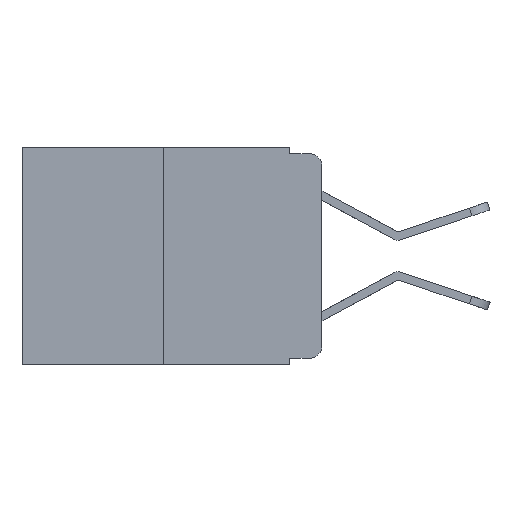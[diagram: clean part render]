
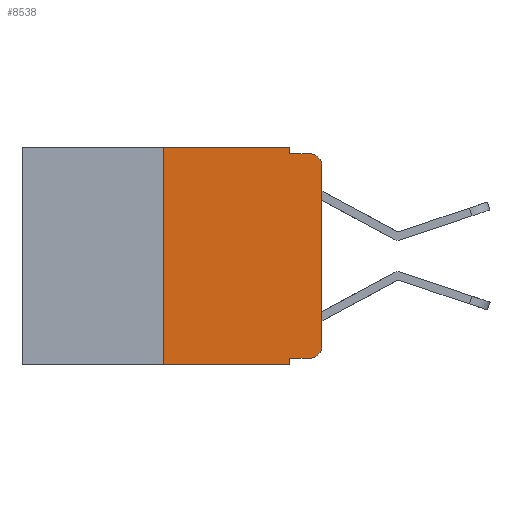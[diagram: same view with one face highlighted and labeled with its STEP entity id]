
A CAD part, left-side view. The second image highlights one B-rep face of the part: STEP entity #8538.
In plain terms, the highlighted planar face has unit normal (-1, 0, 0).
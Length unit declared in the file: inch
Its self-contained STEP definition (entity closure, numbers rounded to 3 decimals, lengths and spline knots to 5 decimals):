
#39 = EDGE_CURVE ( 'NONE', #12802, #1607, #10376, .T. ) ;
#123 = ORIENTED_EDGE ( 'NONE', *, *, #5390, .F. ) ;
#180 = ORIENTED_EDGE ( 'NONE', *, *, #4472, .F. ) ;
#557 = LINE ( 'NONE', #7894, #12925 ) ;
#596 = DIRECTION ( 'NONE',  ( 0., 0., -1. ) ) ;
#652 = LINE ( 'NONE', #930, #7725 ) ;
#930 = CARTESIAN_POINT ( 'NONE',  ( 0., 0.473, -0.343 ) ) ;
#1021 = DIRECTION ( 'NONE',  ( -1., 0., 0. ) ) ;
#1055 = EDGE_CURVE ( 'NONE', #1607, #8877, #1795, .T. ) ;
#1063 = DIRECTION ( 'NONE',  ( 0., 0., 1. ) ) ;
#1137 = CARTESIAN_POINT ( 'NONE',  ( 0., 0.051, -0.343 ) ) ;
#1158 = EDGE_CURVE ( 'NONE', #9367, #1468, #9907, .T. ) ;
#1468 = VERTEX_POINT ( 'NONE', #4644 ) ;
#1482 = VERTEX_POINT ( 'NONE', #1757 ) ;
#1556 = CARTESIAN_POINT ( 'NONE',  ( 0., 0.051, 0. ) ) ;
#1607 = VERTEX_POINT ( 'NONE', #6348 ) ;
#1757 = CARTESIAN_POINT ( 'NONE',  ( 0., 0.25, 0. ) ) ;
#1795 = CIRCLE ( 'NONE', #2024, 0.02 ) ;
#1872 = ORIENTED_EDGE ( 'NONE', *, *, #1055, .T. ) ;
#1900 = VECTOR ( 'NONE', #13041, 39.37008 ) ;
#2024 = AXIS2_PLACEMENT_3D ( 'NONE', #3216, #1021, #5986 ) ;
#2166 = CARTESIAN_POINT ( 'NONE',  ( 0., 0., 0. ) ) ;
#2425 = VERTEX_POINT ( 'NONE', #8123 ) ;
#2855 = DIRECTION ( 'NONE',  ( 0., 0., 1. ) ) ;
#3163 = AXIS2_PLACEMENT_3D ( 'NONE', #7891, #5047, #3957 ) ;
#3193 = EDGE_CURVE ( 'NONE', #12221, #12802, #10938, .T. ) ;
#3216 = CARTESIAN_POINT ( 'NONE',  ( 0., 0.02, -0.03 ) ) ;
#3220 = VECTOR ( 'NONE', #2855, 39.37008 ) ;
#3554 = DIRECTION ( 'NONE',  ( 0., -1., 0. ) ) ;
#3957 = DIRECTION ( 'NONE',  ( 0., 0., -1. ) ) ;
#3971 = ORIENTED_EDGE ( 'NONE', *, *, #39, .T. ) ;
#4472 = EDGE_CURVE ( 'NONE', #1482, #9367, #13350, .T. ) ;
#4633 = CARTESIAN_POINT ( 'NONE',  ( 0., 0.02, -0.01 ) ) ;
#4644 = CARTESIAN_POINT ( 'NONE',  ( 0., 0.051, -0.01 ) ) ;
#5008 = EDGE_CURVE ( 'NONE', #2425, #1482, #6988, .T. ) ;
#5047 = DIRECTION ( 'NONE',  ( -1., 0., 0. ) ) ;
#5390 = EDGE_CURVE ( 'NONE', #5805, #10921, #9148, .T. ) ;
#5736 = EDGE_CURVE ( 'NONE', #5805, #12221, #557, .T. ) ;
#5805 = VERTEX_POINT ( 'NONE', #12883 ) ;
#5837 = DIRECTION ( 'NONE',  ( 0., -1., 0. ) ) ;
#5986 = DIRECTION ( 'NONE',  ( 0., 0., -1. ) ) ;
#6006 = VECTOR ( 'NONE', #10062, 39.37008 ) ;
#6121 = CARTESIAN_POINT ( 'NONE',  ( 0., 0.02, -0.333 ) ) ;
#6348 = CARTESIAN_POINT ( 'NONE',  ( 0., 0., -0.03 ) ) ;
#6764 = DIRECTION ( 'NONE',  ( 1., 0., 0. ) ) ;
#6841 = CARTESIAN_POINT ( 'NONE',  ( 0., 0.051, 0. ) ) ;
#6964 = VECTOR ( 'NONE', #1063, 39.37008 ) ;
#6988 = LINE ( 'NONE', #13122, #3220 ) ;
#7581 = CARTESIAN_POINT ( 'NONE',  ( 0., 0., -0.313 ) ) ;
#7589 = ORIENTED_EDGE ( 'NONE', *, *, #5736, .T. ) ;
#7725 = VECTOR ( 'NONE', #9076, 39.37008 ) ;
#7891 = CARTESIAN_POINT ( 'NONE',  ( 0., 0.02, -0.313 ) ) ;
#7894 = CARTESIAN_POINT ( 'NONE',  ( 0., 0.051, -0.333 ) ) ;
#7932 = CARTESIAN_POINT ( 'NONE',  ( 0., 0.051, 0. ) ) ;
#8069 = VECTOR ( 'NONE', #5837, 39.37008 ) ;
#8078 = ORIENTED_EDGE ( 'NONE', *, *, #3193, .T. ) ;
#8123 = CARTESIAN_POINT ( 'NONE',  ( 0., 0.25, -0.343 ) ) ;
#8281 = EDGE_CURVE ( 'NONE', #1468, #8877, #12310, .T. ) ;
#8538 = ADVANCED_FACE ( 'NONE', ( #8812 ), #10647, .F. ) ;
#8812 = FACE_OUTER_BOUND ( 'NONE', #10488, .T. ) ;
#8877 = VERTEX_POINT ( 'NONE', #4633 ) ;
#9076 = DIRECTION ( 'NONE',  ( 0., -1., 0. ) ) ;
#9148 = LINE ( 'NONE', #6841, #1900 ) ;
#9367 = VERTEX_POINT ( 'NONE', #1556 ) ;
#9841 = ORIENTED_EDGE ( 'NONE', *, *, #8281, .F. ) ;
#9891 = DIRECTION ( 'NONE',  ( 0., 0., -1. ) ) ;
#9907 = LINE ( 'NONE', #7932, #11315 ) ;
#10062 = DIRECTION ( 'NONE',  ( 0., -1., 0. ) ) ;
#10206 = CARTESIAN_POINT ( 'NONE',  ( 0., 0.473, 0. ) ) ;
#10376 = LINE ( 'NONE', #2166, #6964 ) ;
#10488 = EDGE_LOOP ( 'NONE', ( #3971, #1872, #9841, #13179, #180, #12294, #11414, #123, #7589, #8078 ) ) ;
#10647 = PLANE ( 'NONE',  #10711 ) ;
#10711 = AXIS2_PLACEMENT_3D ( 'NONE', #11888, #6764, #9891 ) ;
#10824 = EDGE_CURVE ( 'NONE', #2425, #10921, #652, .T. ) ;
#10921 = VERTEX_POINT ( 'NONE', #1137 ) ;
#10938 = CIRCLE ( 'NONE', #3163, 0.02 ) ;
#10973 = CARTESIAN_POINT ( 'NONE',  ( 0., 0.051, -0.01 ) ) ;
#11315 = VECTOR ( 'NONE', #596, 39.37008 ) ;
#11414 = ORIENTED_EDGE ( 'NONE', *, *, #10824, .T. ) ;
#11888 = CARTESIAN_POINT ( 'NONE',  ( 0., 0.473, 0. ) ) ;
#12221 = VERTEX_POINT ( 'NONE', #6121 ) ;
#12294 = ORIENTED_EDGE ( 'NONE', *, *, #5008, .F. ) ;
#12310 = LINE ( 'NONE', #10973, #8069 ) ;
#12802 = VERTEX_POINT ( 'NONE', #7581 ) ;
#12883 = CARTESIAN_POINT ( 'NONE',  ( 0., 0.051, -0.333 ) ) ;
#12925 = VECTOR ( 'NONE', #3554, 39.37008 ) ;
#13041 = DIRECTION ( 'NONE',  ( 0., 0., -1. ) ) ;
#13122 = CARTESIAN_POINT ( 'NONE',  ( 0., 0.25, 0. ) ) ;
#13179 = ORIENTED_EDGE ( 'NONE', *, *, #1158, .F. ) ;
#13350 = LINE ( 'NONE', #10206, #6006 ) ;
